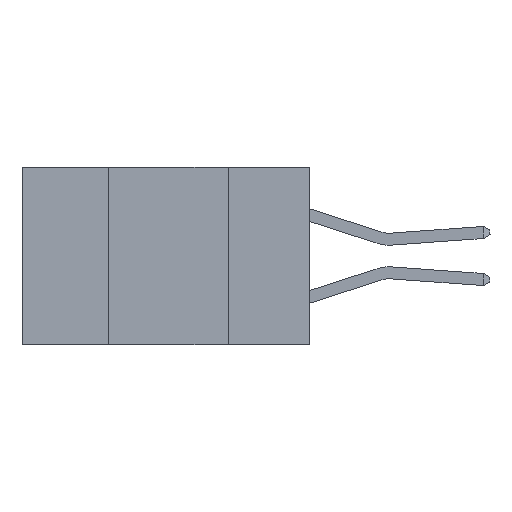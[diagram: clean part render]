
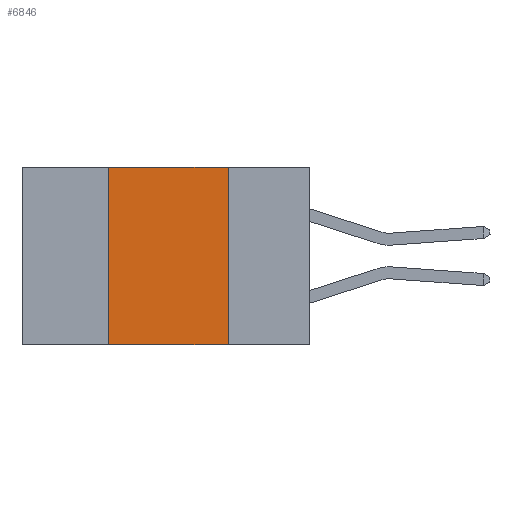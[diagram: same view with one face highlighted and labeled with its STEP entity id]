
A CAD part, left-side view. The second image highlights one B-rep face of the part: STEP entity #6846.
In plain terms, the highlighted planar face has unit normal (-1, 0, 0).
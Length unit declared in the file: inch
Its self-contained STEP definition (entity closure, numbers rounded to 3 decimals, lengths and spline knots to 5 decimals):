
#681 = CARTESIAN_POINT ( 'NONE',  ( 0., 0.17, 0. ) ) ;
#869 = VERTEX_POINT ( 'NONE', #681 ) ;
#1085 = DIRECTION ( 'NONE',  ( 0., 0., 1. ) ) ;
#1830 = VECTOR ( 'NONE', #13392, 39.37008 ) ;
#1879 = CARTESIAN_POINT ( 'NONE',  ( 0., 0.6, -0.37 ) ) ;
#1884 = EDGE_CURVE ( 'NONE', #12679, #16749, #16043, .T. ) ;
#1895 = ORIENTED_EDGE ( 'NONE', *, *, #4046, .F. ) ;
#2132 = CARTESIAN_POINT ( 'NONE',  ( 0., 0.42, 0. ) ) ;
#3117 = DIRECTION ( 'NONE',  ( 1., 0., 0. ) ) ;
#3271 = LINE ( 'NONE', #8759, #8440 ) ;
#3446 = DIRECTION ( 'NONE',  ( 0., -1., 0. ) ) ;
#4046 = EDGE_CURVE ( 'NONE', #869, #16749, #10473, .T. ) ;
#4315 = VERTEX_POINT ( 'NONE', #2132 ) ;
#4549 = PLANE ( 'NONE',  #15452 ) ;
#4722 = ORIENTED_EDGE ( 'NONE', *, *, #1884, .T. ) ;
#5031 = CARTESIAN_POINT ( 'NONE',  ( 0., 0.17, -0.37 ) ) ;
#5147 = CARTESIAN_POINT ( 'NONE',  ( 0., 0.42, 0. ) ) ;
#5869 = CARTESIAN_POINT ( 'NONE',  ( 0., 0.6, 0. ) ) ;
#6846 = ADVANCED_FACE ( 'NONE', ( #12127 ), #4549, .F. ) ;
#6954 = EDGE_CURVE ( 'NONE', #4315, #869, #3271, .T. ) ;
#7265 = DIRECTION ( 'NONE',  ( 0., 0., -1. ) ) ;
#8440 = VECTOR ( 'NONE', #14367, 39.37008 ) ;
#8759 = CARTESIAN_POINT ( 'NONE',  ( 0., 0.6, 0. ) ) ;
#9046 = EDGE_CURVE ( 'NONE', #12679, #4315, #16511, .T. ) ;
#9146 = VECTOR ( 'NONE', #3446, 39.37008 ) ;
#9499 = EDGE_LOOP ( 'NONE', ( #1895, #13650, #12926, #4722 ) ) ;
#9648 = VECTOR ( 'NONE', #1085, 39.37008 ) ;
#10473 = LINE ( 'NONE', #16108, #1830 ) ;
#12127 = FACE_OUTER_BOUND ( 'NONE', #9499, .T. ) ;
#12679 = VERTEX_POINT ( 'NONE', #15412 ) ;
#12926 = ORIENTED_EDGE ( 'NONE', *, *, #9046, .F. ) ;
#13392 = DIRECTION ( 'NONE',  ( 0., 0., -1. ) ) ;
#13650 = ORIENTED_EDGE ( 'NONE', *, *, #6954, .F. ) ;
#14367 = DIRECTION ( 'NONE',  ( 0., -1., 0. ) ) ;
#15412 = CARTESIAN_POINT ( 'NONE',  ( 0., 0.42, -0.37 ) ) ;
#15452 = AXIS2_PLACEMENT_3D ( 'NONE', #5869, #3117, #7265 ) ;
#16043 = LINE ( 'NONE', #1879, #9146 ) ;
#16108 = CARTESIAN_POINT ( 'NONE',  ( 0., 0.17, 0. ) ) ;
#16511 = LINE ( 'NONE', #5147, #9648 ) ;
#16749 = VERTEX_POINT ( 'NONE', #5031 ) ;
